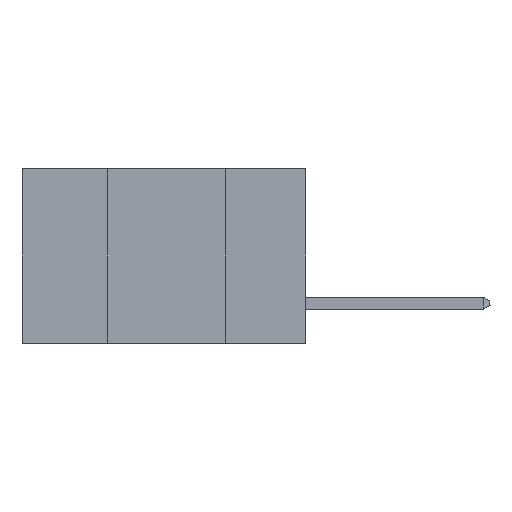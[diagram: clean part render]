
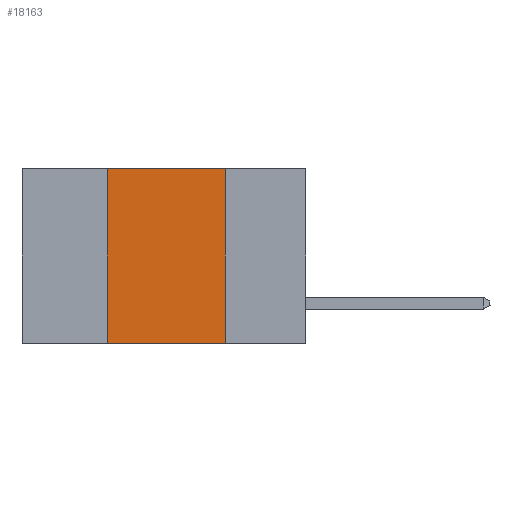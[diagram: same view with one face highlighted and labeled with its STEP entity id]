
A CAD part, left-side view. The second image highlights one B-rep face of the part: STEP entity #18163.
In plain terms, the highlighted planar face has unit normal (-1, 0, 0).
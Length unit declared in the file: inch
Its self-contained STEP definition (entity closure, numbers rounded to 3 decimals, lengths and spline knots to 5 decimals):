
#1509 = LINE ( 'NONE', #8254, #2832 ) ;
#2832 = VECTOR ( 'NONE', #4166, 39.37008 ) ;
#3801 = LINE ( 'NONE', #22233, #5774 ) ;
#4166 = DIRECTION ( 'NONE',  ( 0., 0., 1. ) ) ;
#5556 = CARTESIAN_POINT ( 'NONE',  ( 0., 0.17, 0. ) ) ;
#5774 = VECTOR ( 'NONE', #13918, 39.37008 ) ;
#7763 = FACE_OUTER_BOUND ( 'NONE', #23477, .T. ) ;
#8254 = CARTESIAN_POINT ( 'NONE',  ( 0., 0.42, 0. ) ) ;
#9144 = ORIENTED_EDGE ( 'NONE', *, *, #24367, .F. ) ;
#9279 = DIRECTION ( 'NONE',  ( 0., -1., 0. ) ) ;
#9658 = VERTEX_POINT ( 'NONE', #5556 ) ;
#10865 = VERTEX_POINT ( 'NONE', #19940 ) ;
#11402 = CARTESIAN_POINT ( 'NONE',  ( 0., 0.17, -0.37 ) ) ;
#13918 = DIRECTION ( 'NONE',  ( 0., -1., 0. ) ) ;
#14355 = LINE ( 'NONE', #21967, #20224 ) ;
#15295 = VECTOR ( 'NONE', #9279, 39.37008 ) ;
#17254 = LINE ( 'NONE', #20104, #15295 ) ;
#18163 = ADVANCED_FACE ( 'NONE', ( #7763 ), #20747, .F. ) ;
#18247 = ORIENTED_EDGE ( 'NONE', *, *, #19703, .F. ) ;
#19453 = VERTEX_POINT ( 'NONE', #21979 ) ;
#19703 = EDGE_CURVE ( 'NONE', #19453, #10865, #1509, .T. ) ;
#19940 = CARTESIAN_POINT ( 'NONE',  ( 0., 0.42, 0. ) ) ;
#19945 = EDGE_CURVE ( 'NONE', #19453, #24170, #3801, .T. ) ;
#19983 = DIRECTION ( 'NONE',  ( 0., 0., -1. ) ) ;
#20104 = CARTESIAN_POINT ( 'NONE',  ( 0., 0.6, 0. ) ) ;
#20224 = VECTOR ( 'NONE', #19983, 39.37008 ) ;
#20250 = ORIENTED_EDGE ( 'NONE', *, *, #24574, .F. ) ;
#20411 = ORIENTED_EDGE ( 'NONE', *, *, #19945, .T. ) ;
#20560 = DIRECTION ( 'NONE',  ( 1., 0., 0. ) ) ;
#20747 = PLANE ( 'NONE',  #21542 ) ;
#21542 = AXIS2_PLACEMENT_3D ( 'NONE', #24777, #20560, #22565 ) ;
#21967 = CARTESIAN_POINT ( 'NONE',  ( 0., 0.17, 0. ) ) ;
#21979 = CARTESIAN_POINT ( 'NONE',  ( 0., 0.42, -0.37 ) ) ;
#22233 = CARTESIAN_POINT ( 'NONE',  ( 0., 0.6, -0.37 ) ) ;
#22565 = DIRECTION ( 'NONE',  ( 0., 0., -1. ) ) ;
#23477 = EDGE_LOOP ( 'NONE', ( #9144, #20250, #18247, #20411 ) ) ;
#24170 = VERTEX_POINT ( 'NONE', #11402 ) ;
#24367 = EDGE_CURVE ( 'NONE', #9658, #24170, #14355, .T. ) ;
#24574 = EDGE_CURVE ( 'NONE', #10865, #9658, #17254, .T. ) ;
#24777 = CARTESIAN_POINT ( 'NONE',  ( 0., 0.6, 0. ) ) ;
